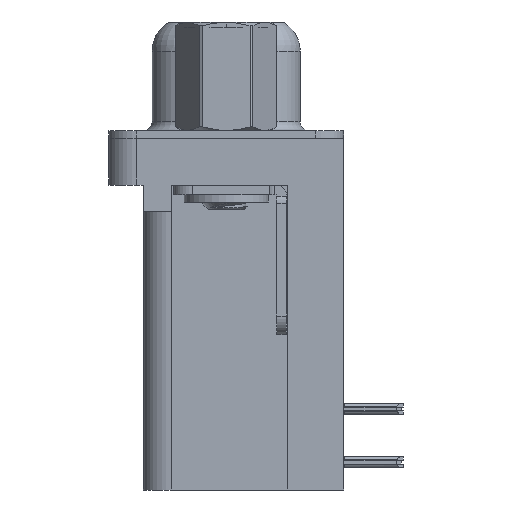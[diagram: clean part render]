
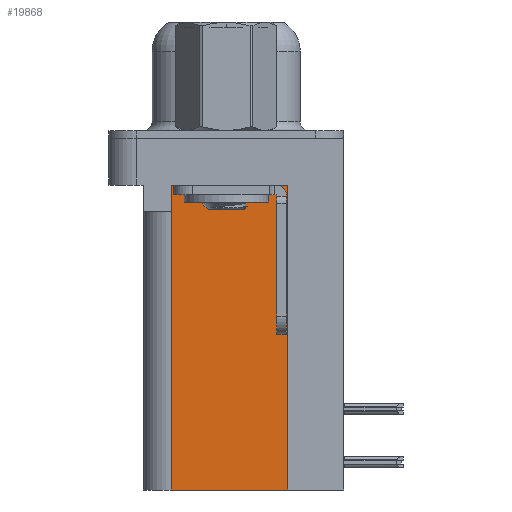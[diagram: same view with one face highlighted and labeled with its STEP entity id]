
A CAD part, left-side view. The second image highlights one B-rep face of the part: STEP entity #19868.
In plain terms, the highlighted planar face has unit normal (-1, 0, 0).
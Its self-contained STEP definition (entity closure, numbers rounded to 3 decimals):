
#4 = LINE ( 'NONE', #15454, #22227 ) ;
#847 = AXIS2_PLACEMENT_3D ( 'NONE', #3380, #6172, #25628 ) ;
#880 = CARTESIAN_POINT ( 'NONE',  ( 3.7, 2.925, -18.76 ) ) ;
#984 = ORIENTED_EDGE ( 'NONE', *, *, #29131, .F. ) ;
#1828 = FACE_OUTER_BOUND ( 'NONE', #31711, .T. ) ;
#3203 = DIRECTION ( 'NONE',  ( 0., 0., 1. ) ) ;
#3380 = CARTESIAN_POINT ( 'NONE',  ( 3.7, -3.295, -18.76 ) ) ;
#3447 = LINE ( 'NONE', #31808, #9915 ) ;
#4399 = ORIENTED_EDGE ( 'NONE', *, *, #32135, .F. ) ;
#4493 = VECTOR ( 'NONE', #23390, 1000. ) ;
#6172 = DIRECTION ( 'NONE',  ( 1., 0., 0. ) ) ;
#6605 = VERTEX_POINT ( 'NONE', #30746 ) ;
#7869 = VERTEX_POINT ( 'NONE', #15841 ) ;
#8946 = CARTESIAN_POINT ( 'NONE',  ( 3.7, -3.295, -18.76 ) ) ;
#9915 = VECTOR ( 'NONE', #34570, 1000. ) ;
#11439 = CARTESIAN_POINT ( 'NONE',  ( 3.7, -3.295, -18.76 ) ) ;
#11459 = ORIENTED_EDGE ( 'NONE', *, *, #22326, .T. ) ;
#11643 = VECTOR ( 'NONE', #3203, 1000. ) ;
#12158 = CARTESIAN_POINT ( 'NONE',  ( 3.7, 2.895, -3.9 ) ) ;
#12554 = LINE ( 'NONE', #8946, #34671 ) ;
#13087 = VERTEX_POINT ( 'NONE', #19676 ) ;
#15454 = CARTESIAN_POINT ( 'NONE',  ( 3.7, 0., -3.9 ) ) ;
#15841 = CARTESIAN_POINT ( 'NONE',  ( 3.7, 2.925, -3.9 ) ) ;
#16885 = CARTESIAN_POINT ( 'NONE',  ( 3.7, 2.925, -18.76 ) ) ;
#19260 = VERTEX_POINT ( 'NONE', #25671 ) ;
#19277 = VECTOR ( 'NONE', #28698, 1000. ) ;
#19676 = CARTESIAN_POINT ( 'NONE',  ( 3.7, -3.295, -2.5 ) ) ;
#19868 = ADVANCED_FACE ( 'NONE', ( #1828 ), #20047, .F. ) ;
#20047 = PLANE ( 'NONE',  #847 ) ;
#20639 = ORIENTED_EDGE ( 'NONE', *, *, #32802, .T. ) ;
#22227 = VECTOR ( 'NONE', #23761, 1000. ) ;
#22326 = EDGE_CURVE ( 'NONE', #13087, #6605, #3447, .T. ) ;
#22453 = CARTESIAN_POINT ( 'NONE',  ( 3.7, 2.895, -3.9 ) ) ;
#22752 = VERTEX_POINT ( 'NONE', #16885 ) ;
#23390 = DIRECTION ( 'NONE',  ( 0., 0., -1. ) ) ;
#23761 = DIRECTION ( 'NONE',  ( 0., 1., 0. ) ) ;
#24830 = ORIENTED_EDGE ( 'NONE', *, *, #29178, .T. ) ;
#25608 = DIRECTION ( 'NONE',  ( 0., 1., 0. ) ) ;
#25628 = DIRECTION ( 'NONE',  ( 0., 1., 0. ) ) ;
#25671 = CARTESIAN_POINT ( 'NONE',  ( 3.7, -3.295, -18.76 ) ) ;
#26591 = ORIENTED_EDGE ( 'NONE', *, *, #31193, .T. ) ;
#26663 = LINE ( 'NONE', #880, #19277 ) ;
#27442 = VERTEX_POINT ( 'NONE', #22453 ) ;
#28698 = DIRECTION ( 'NONE',  ( 0., 0., 1. ) ) ;
#29131 = EDGE_CURVE ( 'NONE', #22752, #7869, #26663, .T. ) ;
#29178 = EDGE_CURVE ( 'NONE', #6605, #27442, #33118, .T. ) ;
#30746 = CARTESIAN_POINT ( 'NONE',  ( 3.7, 2.895, -2.5 ) ) ;
#31193 = EDGE_CURVE ( 'NONE', #27442, #7869, #4, .T. ) ;
#31711 = EDGE_LOOP ( 'NONE', ( #11459, #24830, #26591, #984, #4399, #20639 ) ) ;
#31808 = CARTESIAN_POINT ( 'NONE',  ( 3.7, -3.295, -2.5 ) ) ;
#32135 = EDGE_CURVE ( 'NONE', #19260, #22752, #12554, .T. ) ;
#32802 = EDGE_CURVE ( 'NONE', #19260, #13087, #33779, .T. ) ;
#33118 = LINE ( 'NONE', #12158, #4493 ) ;
#33779 = LINE ( 'NONE', #11439, #11643 ) ;
#34570 = DIRECTION ( 'NONE',  ( 0., 1., 0. ) ) ;
#34671 = VECTOR ( 'NONE', #25608, 1000. ) ;
